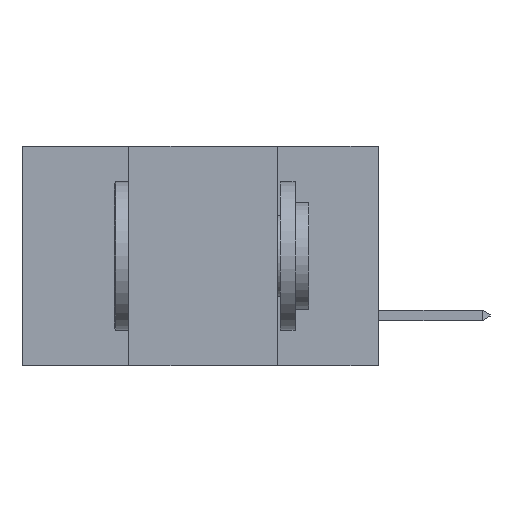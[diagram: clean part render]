
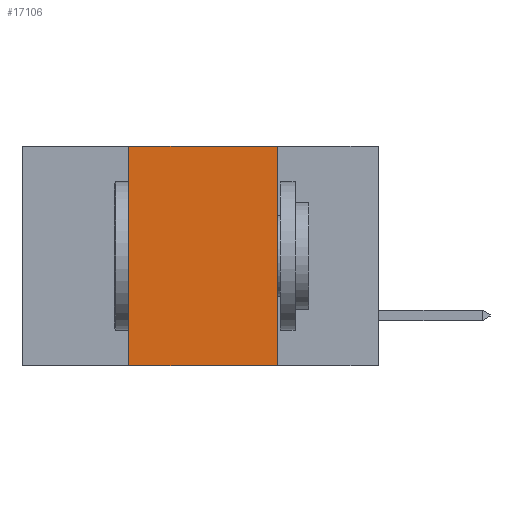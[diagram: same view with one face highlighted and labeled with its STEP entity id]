
A CAD part, left-side view. The second image highlights one B-rep face of the part: STEP entity #17106.
In plain terms, the highlighted planar face has unit normal (-1, 0, 0).
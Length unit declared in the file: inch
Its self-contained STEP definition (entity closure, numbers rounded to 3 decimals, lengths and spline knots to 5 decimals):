
#187 = CARTESIAN_POINT ( 'NONE',  ( 0., 0.42, -0.37 ) ) ;
#1471 = VECTOR ( 'NONE', #22705, 39.37008 ) ;
#3507 = CARTESIAN_POINT ( 'NONE',  ( 0., 0.17, 0. ) ) ;
#3618 = EDGE_CURVE ( 'NONE', #16203, #16198, #18926, .T. ) ;
#4328 = LINE ( 'NONE', #20691, #9173 ) ;
#5715 = VECTOR ( 'NONE', #6164, 39.37008 ) ;
#6164 = DIRECTION ( 'NONE',  ( 0., -1., 0. ) ) ;
#6589 = CARTESIAN_POINT ( 'NONE',  ( 0., 0.6, 0. ) ) ;
#7704 = ORIENTED_EDGE ( 'NONE', *, *, #3618, .F. ) ;
#7898 = AXIS2_PLACEMENT_3D ( 'NONE', #20373, #22074, #11542 ) ;
#7939 = PLANE ( 'NONE',  #7898 ) ;
#8290 = CARTESIAN_POINT ( 'NONE',  ( 0., 0.42, 0. ) ) ;
#8624 = CARTESIAN_POINT ( 'NONE',  ( 0., 0.6, -0.37 ) ) ;
#9112 = VECTOR ( 'NONE', #22328, 39.37008 ) ;
#9173 = VECTOR ( 'NONE', #17231, 39.37008 ) ;
#10339 = VERTEX_POINT ( 'NONE', #187 ) ;
#11542 = DIRECTION ( 'NONE',  ( 0., 0., -1. ) ) ;
#13100 = EDGE_CURVE ( 'NONE', #10339, #19083, #20417, .T. ) ;
#16198 = VERTEX_POINT ( 'NONE', #3507 ) ;
#16203 = VERTEX_POINT ( 'NONE', #17889 ) ;
#16974 = FACE_OUTER_BOUND ( 'NONE', #22253, .T. ) ;
#17106 = ADVANCED_FACE ( 'NONE', ( #16974 ), #7939, .F. ) ;
#17231 = DIRECTION ( 'NONE',  ( 0., 0., -1. ) ) ;
#17244 = ORIENTED_EDGE ( 'NONE', *, *, #21746, .F. ) ;
#17889 = CARTESIAN_POINT ( 'NONE',  ( 0., 0.42, 0. ) ) ;
#17964 = CARTESIAN_POINT ( 'NONE',  ( 0., 0.17, -0.37 ) ) ;
#18926 = LINE ( 'NONE', #6589, #5715 ) ;
#19083 = VERTEX_POINT ( 'NONE', #17964 ) ;
#19495 = EDGE_CURVE ( 'NONE', #16198, #19083, #4328, .T. ) ;
#20373 = CARTESIAN_POINT ( 'NONE',  ( 0., 0.6, 0. ) ) ;
#20417 = LINE ( 'NONE', #8624, #1471 ) ;
#20691 = CARTESIAN_POINT ( 'NONE',  ( 0., 0.17, 0. ) ) ;
#21274 = ORIENTED_EDGE ( 'NONE', *, *, #19495, .F. ) ;
#21746 = EDGE_CURVE ( 'NONE', #10339, #16203, #22596, .T. ) ;
#22074 = DIRECTION ( 'NONE',  ( 1., 0., 0. ) ) ;
#22253 = EDGE_LOOP ( 'NONE', ( #21274, #7704, #17244, #22875 ) ) ;
#22328 = DIRECTION ( 'NONE',  ( 0., 0., 1. ) ) ;
#22596 = LINE ( 'NONE', #8290, #9112 ) ;
#22705 = DIRECTION ( 'NONE',  ( 0., -1., 0. ) ) ;
#22875 = ORIENTED_EDGE ( 'NONE', *, *, #13100, .T. ) ;
